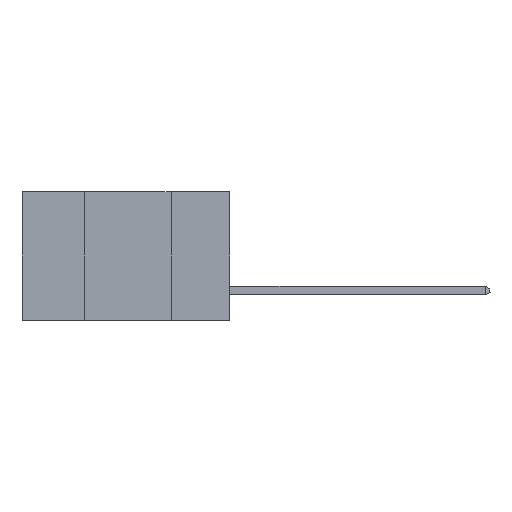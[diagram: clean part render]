
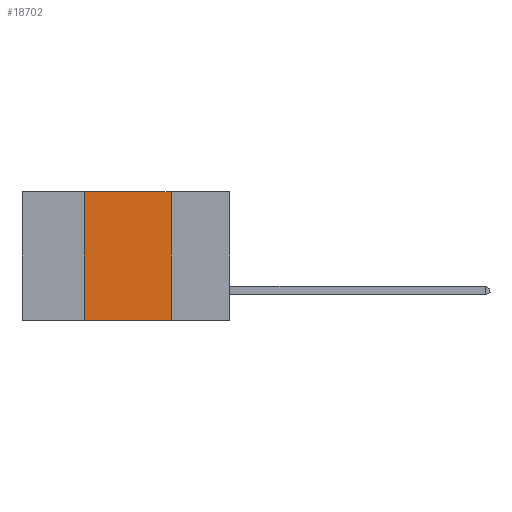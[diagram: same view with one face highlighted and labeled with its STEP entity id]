
A CAD part, left-side view. The second image highlights one B-rep face of the part: STEP entity #18702.
In plain terms, the highlighted planar face has unit normal (-1, 0, 0).
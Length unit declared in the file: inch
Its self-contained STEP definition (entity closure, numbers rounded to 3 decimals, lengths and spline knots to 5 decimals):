
#2035 = CARTESIAN_POINT ( 'NONE',  ( 0., 0.42, 0. ) ) ;
#2277 = CARTESIAN_POINT ( 'NONE',  ( 0., 0.17, 0. ) ) ;
#2584 = LINE ( 'NONE', #3615, #26894 ) ;
#2698 = VERTEX_POINT ( 'NONE', #2277 ) ;
#3615 = CARTESIAN_POINT ( 'NONE',  ( 0., 0.17, 0. ) ) ;
#3737 = EDGE_CURVE ( 'NONE', #14831, #2698, #6858, .T. ) ;
#4221 = CARTESIAN_POINT ( 'NONE',  ( 0., 0.6, -0.37 ) ) ;
#5752 = DIRECTION ( 'NONE',  ( 0., 0., -1. ) ) ;
#6858 = LINE ( 'NONE', #10936, #14227 ) ;
#7296 = CARTESIAN_POINT ( 'NONE',  ( 0., 0.42, 0. ) ) ;
#7520 = ORIENTED_EDGE ( 'NONE', *, *, #27474, .T. ) ;
#8008 = DIRECTION ( 'NONE',  ( 0., 0., -1. ) ) ;
#8108 = PLANE ( 'NONE',  #16311 ) ;
#9989 = VERTEX_POINT ( 'NONE', #18996 ) ;
#10091 = DIRECTION ( 'NONE',  ( 1., 0., 0. ) ) ;
#10936 = CARTESIAN_POINT ( 'NONE',  ( 0., 0.6, 0. ) ) ;
#10939 = ORIENTED_EDGE ( 'NONE', *, *, #17938, .F. ) ;
#11355 = DIRECTION ( 'NONE',  ( 0., 0., 1. ) ) ;
#13867 = CARTESIAN_POINT ( 'NONE',  ( 0., 0.42, -0.37 ) ) ;
#14227 = VECTOR ( 'NONE', #16072, 39.37008 ) ;
#14831 = VERTEX_POINT ( 'NONE', #7296 ) ;
#14982 = VECTOR ( 'NONE', #30177, 39.37008 ) ;
#16072 = DIRECTION ( 'NONE',  ( 0., -1., 0. ) ) ;
#16311 = AXIS2_PLACEMENT_3D ( 'NONE', #22145, #10091, #8008 ) ;
#17492 = EDGE_CURVE ( 'NONE', #18459, #14831, #27654, .T. ) ;
#17938 = EDGE_CURVE ( 'NONE', #2698, #9989, #2584, .T. ) ;
#18285 = ORIENTED_EDGE ( 'NONE', *, *, #17492, .F. ) ;
#18459 = VERTEX_POINT ( 'NONE', #13867 ) ;
#18702 = ADVANCED_FACE ( 'NONE', ( #26714 ), #8108, .F. ) ;
#18996 = CARTESIAN_POINT ( 'NONE',  ( 0., 0.17, -0.37 ) ) ;
#19386 = LINE ( 'NONE', #4221, #14982 ) ;
#22022 = ORIENTED_EDGE ( 'NONE', *, *, #3737, .F. ) ;
#22145 = CARTESIAN_POINT ( 'NONE',  ( 0., 0.6, 0. ) ) ;
#23661 = EDGE_LOOP ( 'NONE', ( #10939, #22022, #18285, #7520 ) ) ;
#25469 = VECTOR ( 'NONE', #11355, 39.37008 ) ;
#26714 = FACE_OUTER_BOUND ( 'NONE', #23661, .T. ) ;
#26894 = VECTOR ( 'NONE', #5752, 39.37008 ) ;
#27474 = EDGE_CURVE ( 'NONE', #18459, #9989, #19386, .T. ) ;
#27654 = LINE ( 'NONE', #2035, #25469 ) ;
#30177 = DIRECTION ( 'NONE',  ( 0., -1., 0. ) ) ;
